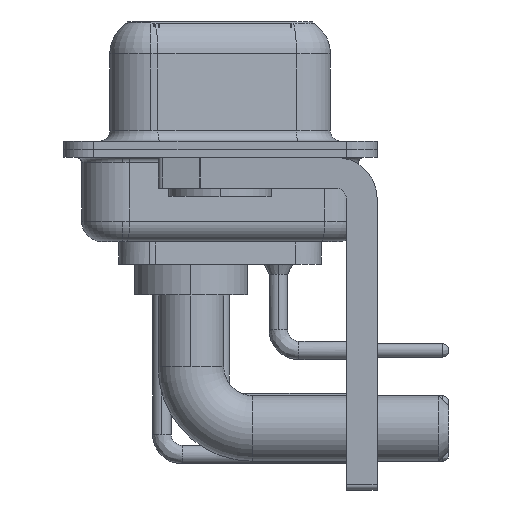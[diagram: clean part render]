
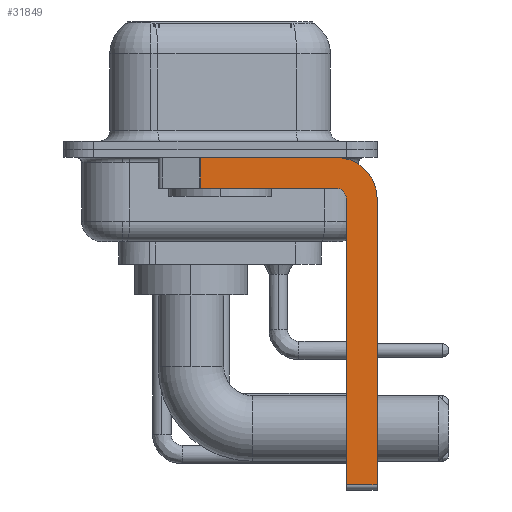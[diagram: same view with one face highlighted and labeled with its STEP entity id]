
A CAD part, left-side view. The second image highlights one B-rep face of the part: STEP entity #31849.
In plain terms, the highlighted planar face has unit normal (-1, 0, 0).
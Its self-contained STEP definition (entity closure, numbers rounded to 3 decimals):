
#10 = ORIENTED_EDGE ( 'NONE', *, *, #21883, .F. ) ;
#712 = VERTEX_POINT ( 'NONE', #23107 ) ;
#983 = ORIENTED_EDGE ( 'NONE', *, *, #10995, .F. ) ;
#1868 = ORIENTED_EDGE ( 'NONE', *, *, #24238, .F. ) ;
#3937 = DIRECTION ( 'NONE',  ( -1., 0., 0. ) ) ;
#4225 = CARTESIAN_POINT ( 'NONE',  ( -2.9, -5.65, -0.4 ) ) ;
#4247 = DIRECTION ( 'NONE',  ( 1., 0., 0. ) ) ;
#4552 = EDGE_CURVE ( 'NONE', #712, #32762, #13261, .T. ) ;
#4755 = CARTESIAN_POINT ( 'NONE',  ( -2.9, -7.65, -2.4 ) ) ;
#4807 = ORIENTED_EDGE ( 'NONE', *, *, #27808, .T. ) ;
#5968 = EDGE_CURVE ( 'NONE', #28860, #15656, #12932, .T. ) ;
#6021 = CARTESIAN_POINT ( 'NONE',  ( -2.9, -5.65, -2.4 ) ) ;
#6633 = ORIENTED_EDGE ( 'NONE', *, *, #4552, .T. ) ;
#6715 = CARTESIAN_POINT ( 'NONE',  ( -2.9, -7.65, -2.4 ) ) ;
#7360 = LINE ( 'NONE', #18252, #13513 ) ;
#7700 = CARTESIAN_POINT ( 'NONE',  ( -2.9, -5.65, -1.9 ) ) ;
#7996 = CARTESIAN_POINT ( 'NONE',  ( -2.9, -6.15, -16.6 ) ) ;
#9738 = DIRECTION ( 'NONE',  ( 0., 0., 1. ) ) ;
#9893 = DIRECTION ( 'NONE',  ( 0., 0., -1. ) ) ;
#10247 = DIRECTION ( 'NONE',  ( 0., 1., 0. ) ) ;
#10573 = CIRCLE ( 'NONE', #17309, 0.5 ) ;
#10995 = EDGE_CURVE ( 'NONE', #24216, #32762, #24107, .T. ) ;
#12932 = LINE ( 'NONE', #7996, #31212 ) ;
#13099 = DIRECTION ( 'NONE',  ( 0., 0., 1. ) ) ;
#13261 = LINE ( 'NONE', #21170, #19301 ) ;
#13408 = AXIS2_PLACEMENT_3D ( 'NONE', #6021, #29750, #30445 ) ;
#13513 = VECTOR ( 'NONE', #15617, 1000. ) ;
#13793 = EDGE_LOOP ( 'NONE', ( #1868, #6633, #983, #10, #15980, #4807, #22553, #21471 ) ) ;
#15163 = VERTEX_POINT ( 'NONE', #23118 ) ;
#15180 = VECTOR ( 'NONE', #9893, 1000. ) ;
#15617 = DIRECTION ( 'NONE',  ( 0., -1., 0. ) ) ;
#15656 = VERTEX_POINT ( 'NONE', #31650 ) ;
#15848 = CARTESIAN_POINT ( 'NONE',  ( -2.9, -5.65, -1.9 ) ) ;
#15980 = ORIENTED_EDGE ( 'NONE', *, *, #5968, .F. ) ;
#16560 = PLANE ( 'NONE',  #13408 ) ;
#17267 = LINE ( 'NONE', #6715, #15180 ) ;
#17309 = AXIS2_PLACEMENT_3D ( 'NONE', #20439, #3937, #9738 ) ;
#18252 = CARTESIAN_POINT ( 'NONE',  ( -2.9, 3., -0.4 ) ) ;
#19079 = DIRECTION ( 'NONE',  ( 0., -1., 0. ) ) ;
#19301 = VECTOR ( 'NONE', #24162, 1000. ) ;
#20439 = CARTESIAN_POINT ( 'NONE',  ( -2.9, -5.65, -2.4 ) ) ;
#21170 = CARTESIAN_POINT ( 'NONE',  ( -2.9, 0.978, -1.9 ) ) ;
#21471 = ORIENTED_EDGE ( 'NONE', *, *, #30073, .F. ) ;
#21883 = EDGE_CURVE ( 'NONE', #15656, #24216, #10573, .T. ) ;
#22086 = VECTOR ( 'NONE', #19079, 1000. ) ;
#22553 = ORIENTED_EDGE ( 'NONE', *, *, #33359, .F. ) ;
#22817 = CIRCLE ( 'NONE', #27294, 2. ) ;
#23107 = CARTESIAN_POINT ( 'NONE',  ( -2.9, 0.978, -0.4 ) ) ;
#23118 = CARTESIAN_POINT ( 'NONE',  ( -2.9, -7.65, -16.35 ) ) ;
#24107 = LINE ( 'NONE', #15848, #27127 ) ;
#24162 = DIRECTION ( 'NONE',  ( 0., 0., -1. ) ) ;
#24216 = VERTEX_POINT ( 'NONE', #7700 ) ;
#24238 = EDGE_CURVE ( 'NONE', #712, #32491, #7360, .T. ) ;
#24363 = LINE ( 'NONE', #30321, #22086 ) ;
#27127 = VECTOR ( 'NONE', #10247, 1000. ) ;
#27294 = AXIS2_PLACEMENT_3D ( 'NONE', #33761, #4247, #28122 ) ;
#27808 = EDGE_CURVE ( 'NONE', #28860, #15163, #24363, .T. ) ;
#28122 = DIRECTION ( 'NONE',  ( 0., 0., -1. ) ) ;
#28860 = VERTEX_POINT ( 'NONE', #30590 ) ;
#28972 = VERTEX_POINT ( 'NONE', #4755 ) ;
#29750 = DIRECTION ( 'NONE',  ( 1., 0., 0. ) ) ;
#30073 = EDGE_CURVE ( 'NONE', #32491, #28972, #22817, .T. ) ;
#30321 = CARTESIAN_POINT ( 'NONE',  ( -2.9, -5.65, -16.35 ) ) ;
#30445 = DIRECTION ( 'NONE',  ( 0., 0., -1. ) ) ;
#30590 = CARTESIAN_POINT ( 'NONE',  ( -2.9, -6.15, -16.35 ) ) ;
#30660 = CARTESIAN_POINT ( 'NONE',  ( -2.9, 0.978, -1.9 ) ) ;
#31212 = VECTOR ( 'NONE', #13099, 1000. ) ;
#31650 = CARTESIAN_POINT ( 'NONE',  ( -2.9, -6.15, -2.4 ) ) ;
#31849 = ADVANCED_FACE ( 'NONE', ( #33072 ), #16560, .F. ) ;
#32491 = VERTEX_POINT ( 'NONE', #4225 ) ;
#32762 = VERTEX_POINT ( 'NONE', #30660 ) ;
#33072 = FACE_OUTER_BOUND ( 'NONE', #13793, .T. ) ;
#33359 = EDGE_CURVE ( 'NONE', #28972, #15163, #17267, .T. ) ;
#33761 = CARTESIAN_POINT ( 'NONE',  ( -2.9, -5.65, -2.4 ) ) ;
